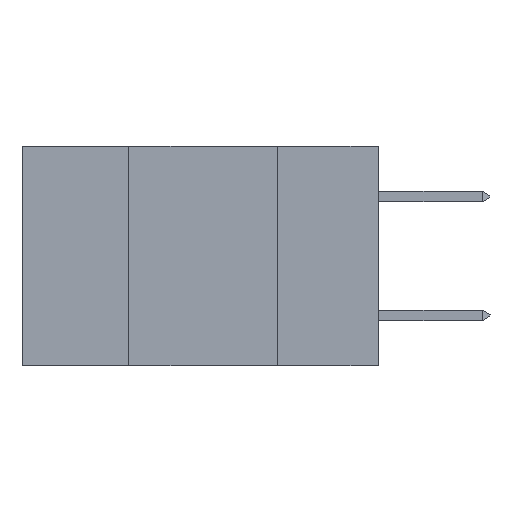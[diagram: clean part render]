
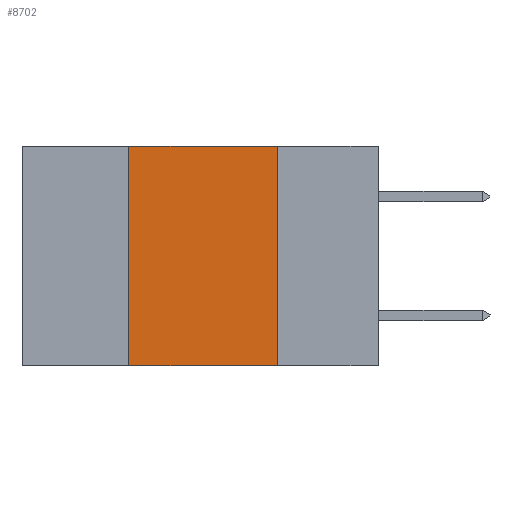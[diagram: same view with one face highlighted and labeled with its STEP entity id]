
A CAD part, left-side view. The second image highlights one B-rep face of the part: STEP entity #8702.
In plain terms, the highlighted planar face has unit normal (-1, 0, 0).
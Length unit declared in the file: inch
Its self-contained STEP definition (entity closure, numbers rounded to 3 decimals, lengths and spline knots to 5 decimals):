
#200 = DIRECTION ( 'NONE',  ( 0., 0., -1. ) ) ;
#1041 = EDGE_CURVE ( 'NONE', #15808, #10588, #15269, .T. ) ;
#1246 = ORIENTED_EDGE ( 'NONE', *, *, #6912, .F. ) ;
#1591 = LINE ( 'NONE', #17844, #14814 ) ;
#2076 = EDGE_CURVE ( 'NONE', #10588, #17206, #9160, .T. ) ;
#3080 = LINE ( 'NONE', #4451, #11576 ) ;
#4387 = VECTOR ( 'NONE', #6099, 39.37008 ) ;
#4451 = CARTESIAN_POINT ( 'NONE',  ( 0., 0.6, -0.37 ) ) ;
#6099 = DIRECTION ( 'NONE',  ( 0., 0., 1. ) ) ;
#6293 = VECTOR ( 'NONE', #15076, 39.37008 ) ;
#6336 = AXIS2_PLACEMENT_3D ( 'NONE', #6994, #8484, #200 ) ;
#6496 = EDGE_CURVE ( 'NONE', #15808, #17830, #3080, .T. ) ;
#6639 = CARTESIAN_POINT ( 'NONE',  ( 0., 0.42, 0. ) ) ;
#6912 = EDGE_CURVE ( 'NONE', #17206, #17830, #1591, .T. ) ;
#6994 = CARTESIAN_POINT ( 'NONE',  ( 0., 0.6, 0. ) ) ;
#8484 = DIRECTION ( 'NONE',  ( 1., 0., 0. ) ) ;
#8594 = DIRECTION ( 'NONE',  ( 0., -1., 0. ) ) ;
#8702 = ADVANCED_FACE ( 'NONE', ( #13456 ), #15048, .F. ) ;
#9160 = LINE ( 'NONE', #16374, #6293 ) ;
#9492 = ORIENTED_EDGE ( 'NONE', *, *, #6496, .T. ) ;
#9502 = ORIENTED_EDGE ( 'NONE', *, *, #1041, .F. ) ;
#10588 = VERTEX_POINT ( 'NONE', #6639 ) ;
#11576 = VECTOR ( 'NONE', #8594, 39.37008 ) ;
#12727 = EDGE_LOOP ( 'NONE', ( #1246, #17435, #9502, #9492 ) ) ;
#12752 = CARTESIAN_POINT ( 'NONE',  ( 0., 0.17, -0.37 ) ) ;
#13456 = FACE_OUTER_BOUND ( 'NONE', #12727, .T. ) ;
#14333 = CARTESIAN_POINT ( 'NONE',  ( 0., 0.42, 0. ) ) ;
#14682 = CARTESIAN_POINT ( 'NONE',  ( 0., 0.17, 0. ) ) ;
#14814 = VECTOR ( 'NONE', #17774, 39.37008 ) ;
#15048 = PLANE ( 'NONE',  #6336 ) ;
#15076 = DIRECTION ( 'NONE',  ( 0., -1., 0. ) ) ;
#15269 = LINE ( 'NONE', #14333, #4387 ) ;
#15808 = VERTEX_POINT ( 'NONE', #17000 ) ;
#16374 = CARTESIAN_POINT ( 'NONE',  ( 0., 0.6, 0. ) ) ;
#17000 = CARTESIAN_POINT ( 'NONE',  ( 0., 0.42, -0.37 ) ) ;
#17206 = VERTEX_POINT ( 'NONE', #14682 ) ;
#17435 = ORIENTED_EDGE ( 'NONE', *, *, #2076, .F. ) ;
#17774 = DIRECTION ( 'NONE',  ( 0., 0., -1. ) ) ;
#17830 = VERTEX_POINT ( 'NONE', #12752 ) ;
#17844 = CARTESIAN_POINT ( 'NONE',  ( 0., 0.17, 0. ) ) ;
